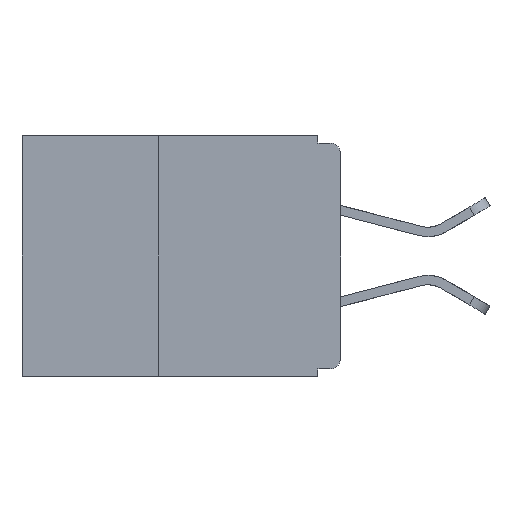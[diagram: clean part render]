
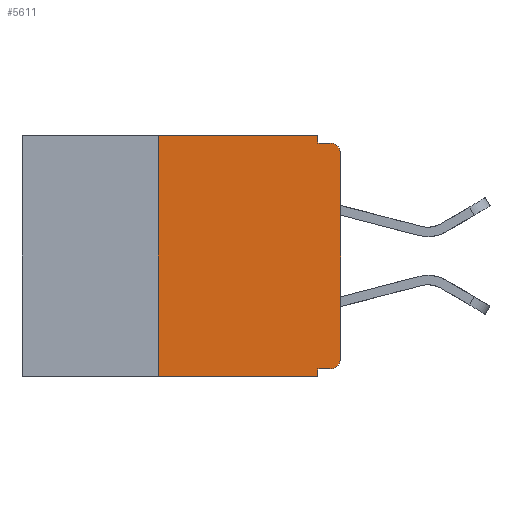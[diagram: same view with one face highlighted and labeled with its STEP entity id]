
A CAD part, left-side view. The second image highlights one B-rep face of the part: STEP entity #5611.
In plain terms, the highlighted planar face has unit normal (-1, 0, 0).
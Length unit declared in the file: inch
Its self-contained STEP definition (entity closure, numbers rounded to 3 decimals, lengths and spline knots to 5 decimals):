
#141 = VERTEX_POINT ( 'NONE', #15249 ) ;
#484 = VERTEX_POINT ( 'NONE', #22394 ) ;
#663 = CARTESIAN_POINT ( 'NONE',  ( 0., 0.015, -0.025 ) ) ;
#900 = CARTESIAN_POINT ( 'NONE',  ( 0., 0.25, -0.33 ) ) ;
#1524 = ORIENTED_EDGE ( 'NONE', *, *, #12754, .F. ) ;
#2139 = ORIENTED_EDGE ( 'NONE', *, *, #7420, .F. ) ;
#2195 = CARTESIAN_POINT ( 'NONE',  ( 0., 0.25, 0. ) ) ;
#2460 = DIRECTION ( 'NONE',  ( 0., 0., -1. ) ) ;
#2547 = DIRECTION ( 'NONE',  ( 0., 0., 1. ) ) ;
#2559 = DIRECTION ( 'NONE',  ( 0., 1., 0. ) ) ;
#2586 = CARTESIAN_POINT ( 'NONE',  ( 0., 0., -0.32 ) ) ;
#2812 = LINE ( 'NONE', #12768, #7550 ) ;
#3038 = LINE ( 'NONE', #11054, #16530 ) ;
#3054 = CARTESIAN_POINT ( 'NONE',  ( 0., 0.031, 0. ) ) ;
#3170 = LINE ( 'NONE', #14915, #6796 ) ;
#3965 = DIRECTION ( 'NONE',  ( 0., -1., 0. ) ) ;
#4004 = VECTOR ( 'NONE', #8004, 39.37008 ) ;
#4203 = VERTEX_POINT ( 'NONE', #2195 ) ;
#4214 = DIRECTION ( 'NONE',  ( 0., 0., -1. ) ) ;
#4245 = CARTESIAN_POINT ( 'NONE',  ( 0., 0.031, -0.33 ) ) ;
#4861 = VECTOR ( 'NONE', #11025, 39.37008 ) ;
#5421 = VERTEX_POINT ( 'NONE', #3054 ) ;
#5556 = ORIENTED_EDGE ( 'NONE', *, *, #8073, .F. ) ;
#5611 = ADVANCED_FACE ( 'NONE', ( #15938 ), #20277, .F. ) ;
#6796 = VECTOR ( 'NONE', #2547, 39.37008 ) ;
#7059 = DIRECTION ( 'NONE',  ( -1., 0., 0. ) ) ;
#7412 = CIRCLE ( 'NONE', #12541, 0.015 ) ;
#7420 = EDGE_CURVE ( 'NONE', #5421, #20642, #18823, .T. ) ;
#7519 = VERTEX_POINT ( 'NONE', #10025 ) ;
#7550 = VECTOR ( 'NONE', #3965, 39.37008 ) ;
#7683 = EDGE_CURVE ( 'NONE', #20642, #14852, #17999, .T. ) ;
#7749 = VECTOR ( 'NONE', #4214, 39.37008 ) ;
#8004 = DIRECTION ( 'NONE',  ( 0., -1., 0. ) ) ;
#8053 = CARTESIAN_POINT ( 'NONE',  ( 0., 0.015, -0.01 ) ) ;
#8073 = EDGE_CURVE ( 'NONE', #19587, #141, #12411, .T. ) ;
#8233 = EDGE_CURVE ( 'NONE', #7519, #19587, #13803, .T. ) ;
#8477 = CARTESIAN_POINT ( 'NONE',  ( 0., 0., -0.025 ) ) ;
#8482 = CARTESIAN_POINT ( 'NONE',  ( 0., 0., -0.01 ) ) ;
#9128 = VECTOR ( 'NONE', #2559, 39.37008 ) ;
#9225 = EDGE_CURVE ( 'NONE', #7519, #484, #7412, .T. ) ;
#9362 = EDGE_LOOP ( 'NONE', ( #20779, #14052, #18884, #2139, #1524, #14360, #18900, #5556, #16765, #19141 ) ) ;
#10025 = CARTESIAN_POINT ( 'NONE',  ( 0., 0.015, -0.32 ) ) ;
#10276 = EDGE_CURVE ( 'NONE', #12988, #141, #17785, .T. ) ;
#10974 = CARTESIAN_POINT ( 'NONE',  ( 0., 0.031, 0. ) ) ;
#11025 = DIRECTION ( 'NONE',  ( 0., 0., -1. ) ) ;
#11054 = CARTESIAN_POINT ( 'NONE',  ( 0., 0.25, -0.33 ) ) ;
#11270 = EDGE_CURVE ( 'NONE', #484, #20237, #3170, .T. ) ;
#11289 = CARTESIAN_POINT ( 'NONE',  ( 0., 0.031, -0.01 ) ) ;
#11556 = CARTESIAN_POINT ( 'NONE',  ( 0., 0.437, -0.33 ) ) ;
#12272 = CARTESIAN_POINT ( 'NONE',  ( 0., 0.031, -0.32 ) ) ;
#12411 = LINE ( 'NONE', #4245, #7749 ) ;
#12541 = AXIS2_PLACEMENT_3D ( 'NONE', #17521, #7059, #19290 ) ;
#12754 = EDGE_CURVE ( 'NONE', #4203, #5421, #2812, .T. ) ;
#12768 = CARTESIAN_POINT ( 'NONE',  ( 0., 0.437, 0. ) ) ;
#12988 = VERTEX_POINT ( 'NONE', #900 ) ;
#13069 = DIRECTION ( 'NONE',  ( -1., 0., 0. ) ) ;
#13192 = VECTOR ( 'NONE', #18560, 39.37008 ) ;
#13803 = LINE ( 'NONE', #2586, #9128 ) ;
#14052 = ORIENTED_EDGE ( 'NONE', *, *, #19860, .T. ) ;
#14360 = ORIENTED_EDGE ( 'NONE', *, *, #14674, .F. ) ;
#14674 = EDGE_CURVE ( 'NONE', #12988, #4203, #3038, .T. ) ;
#14852 = VERTEX_POINT ( 'NONE', #8053 ) ;
#14915 = CARTESIAN_POINT ( 'NONE',  ( 0., 0., 0. ) ) ;
#15249 = CARTESIAN_POINT ( 'NONE',  ( 0., 0.031, -0.33 ) ) ;
#15414 = AXIS2_PLACEMENT_3D ( 'NONE', #20679, #20658, #15687 ) ;
#15687 = DIRECTION ( 'NONE',  ( 0., 0., -1. ) ) ;
#15938 = FACE_OUTER_BOUND ( 'NONE', #9362, .T. ) ;
#16530 = VECTOR ( 'NONE', #19770, 39.37008 ) ;
#16765 = ORIENTED_EDGE ( 'NONE', *, *, #8233, .F. ) ;
#16900 = AXIS2_PLACEMENT_3D ( 'NONE', #663, #13069, #2460 ) ;
#17352 = CIRCLE ( 'NONE', #16900, 0.015 ) ;
#17521 = CARTESIAN_POINT ( 'NONE',  ( 0., 0.015, -0.305 ) ) ;
#17785 = LINE ( 'NONE', #11556, #13192 ) ;
#17999 = LINE ( 'NONE', #8482, #4004 ) ;
#18560 = DIRECTION ( 'NONE',  ( 0., -1., 0. ) ) ;
#18823 = LINE ( 'NONE', #10974, #4861 ) ;
#18884 = ORIENTED_EDGE ( 'NONE', *, *, #7683, .F. ) ;
#18900 = ORIENTED_EDGE ( 'NONE', *, *, #10276, .T. ) ;
#19141 = ORIENTED_EDGE ( 'NONE', *, *, #9225, .T. ) ;
#19290 = DIRECTION ( 'NONE',  ( 0., 0., -1. ) ) ;
#19587 = VERTEX_POINT ( 'NONE', #12272 ) ;
#19770 = DIRECTION ( 'NONE',  ( 0., 0., 1. ) ) ;
#19860 = EDGE_CURVE ( 'NONE', #20237, #14852, #17352, .T. ) ;
#20237 = VERTEX_POINT ( 'NONE', #8477 ) ;
#20277 = PLANE ( 'NONE',  #15414 ) ;
#20642 = VERTEX_POINT ( 'NONE', #11289 ) ;
#20658 = DIRECTION ( 'NONE',  ( 1., 0., 0. ) ) ;
#20679 = CARTESIAN_POINT ( 'NONE',  ( 0., 0.437, 0. ) ) ;
#20779 = ORIENTED_EDGE ( 'NONE', *, *, #11270, .T. ) ;
#22394 = CARTESIAN_POINT ( 'NONE',  ( 0., 0., -0.305 ) ) ;
